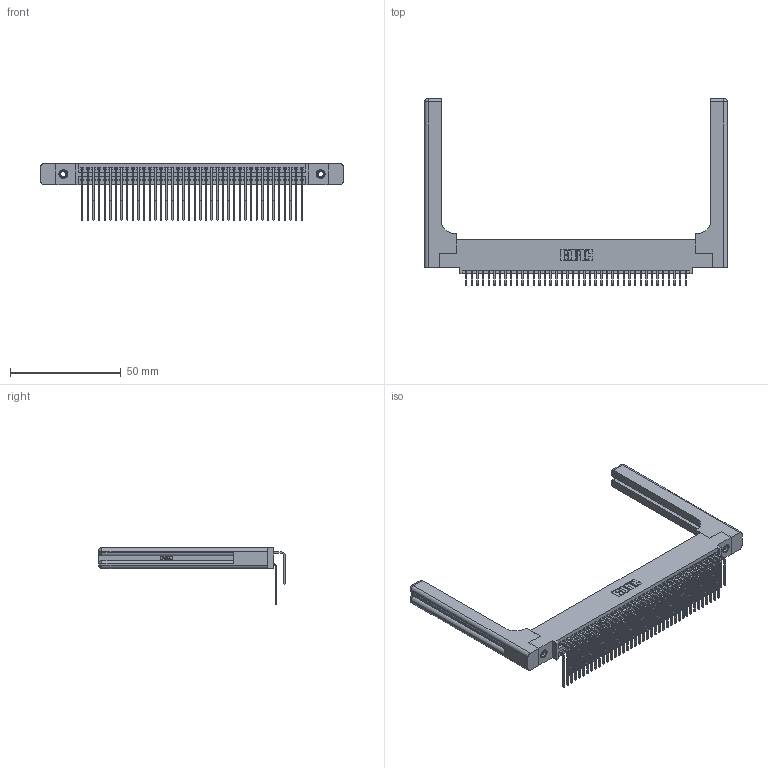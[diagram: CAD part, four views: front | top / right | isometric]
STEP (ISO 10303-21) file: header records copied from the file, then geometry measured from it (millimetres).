
FILE_DESCRIPTION (( 'STEP AP203' ), '1' );
FILE_NAME ('345-080-559-558.STEP', '2019-10-31T20:57:40', ( '' ), ( '' ), 'SwSTEP 2.0', 'SolidWorks 2016', '' );
FILE_SCHEMA (( 'CONFIG_CONTROL_DESIGN' ));
Length unit declared in the file: inch
Products named in the file (6): 345-292-001_559 Tail - 2; 345-220-058_345-220-058; 345-292-001_558 559 Tail - 1; 345-080-559-558; 345 Part_0.110 Offset - 0.156 Dia-TH; 345-250-001_345-250-001-102
Assembly tree (85 placements, depth 2):
  345-080-559-558
    345 Part_0.110 Offset - 0.156 Dia-TH
    345-292-001_558 559 Tail - 1  x40
    345-292-001_559 Tail - 2  x40
    345-250-001_345-250-001-102  x2
    345-220-058_345-220-058  x2
Bounding box: 136.63 x 84.32 x 25.53 mm (x, y, z)
Volume: 22116.7 mm3; surface area: 27447.7 mm2
Topology: 85 solids, 85 shells, 4546 faces, 13419 edges, 8818 vertices
Faces by surface type: plane 3032, cylinder 1454, bspline 36, cone 12, sphere 8, torus 4
Entity records: 38620 total; most frequent: CARTESIAN_POINT 7516, ORIENTED_EDGE 6196, DIRECTION 5534, EDGE_CURVE 3098, VECTOR 2674, LINE 2674, VERTEX_POINT 2054, AXIS2_PLACEMENT_3D 1430
